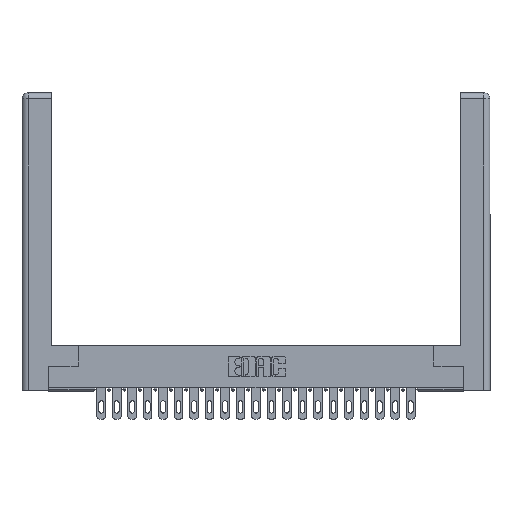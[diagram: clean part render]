
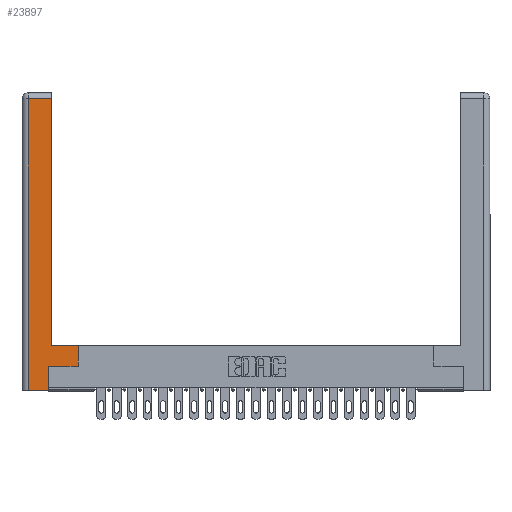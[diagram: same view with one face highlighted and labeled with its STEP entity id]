
A CAD part, top view. The second image highlights one B-rep face of the part: STEP entity #23897.
In plain terms, the highlighted planar face has unit normal (0, 0, 1).
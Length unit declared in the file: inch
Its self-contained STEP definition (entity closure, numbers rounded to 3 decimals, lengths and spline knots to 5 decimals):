
#56 = VERTEX_POINT ( 'NONE', #20512 ) ;
#331 = VERTEX_POINT ( 'NONE', #8046 ) ;
#447 = CARTESIAN_POINT ( 'NONE',  ( 0.565, 0.45, 0. ) ) ;
#482 = DIRECTION ( 'NONE',  ( 1., 0., 0. ) ) ;
#1216 = LINE ( 'NONE', #9743, #21261 ) ;
#1242 = CARTESIAN_POINT ( 'NONE',  ( 0.0615, 0., 0. ) ) ;
#1908 = EDGE_CURVE ( 'NONE', #331, #20292, #1216, .T. ) ;
#2259 = EDGE_CURVE ( 'NONE', #56, #16044, #23649, .T. ) ;
#2701 = DIRECTION ( 'NONE',  ( -1., 0., 0. ) ) ;
#2729 = CARTESIAN_POINT ( 'NONE',  ( 0.0615, 0., 0. ) ) ;
#3639 = EDGE_CURVE ( 'NONE', #20161, #331, #24363, .T. ) ;
#4570 = LINE ( 'NONE', #18500, #14320 ) ;
#4884 = DIRECTION ( 'NONE',  ( 0., 1., 0. ) ) ;
#5292 = DIRECTION ( 'NONE',  ( -1., 0., 0. ) ) ;
#5358 = CARTESIAN_POINT ( 'NONE',  ( 0.0615, 2.94, 0. ) ) ;
#5821 = DIRECTION ( 'NONE',  ( 1., 0., 0. ) ) ;
#6490 = EDGE_LOOP ( 'NONE', ( #11118, #15841, #23320, #9369, #12579, #12570, #23972, #16701 ) ) ;
#6543 = CARTESIAN_POINT ( 'NONE',  ( 0., 0., 0. ) ) ;
#7590 = AXIS2_PLACEMENT_3D ( 'NONE', #6543, #14395, #2701 ) ;
#7880 = VECTOR ( 'NONE', #23703, 39.37008 ) ;
#8046 = CARTESIAN_POINT ( 'NONE',  ( 0.265, 0., 0. ) ) ;
#8336 = VECTOR ( 'NONE', #5821, 39.37008 ) ;
#8548 = VECTOR ( 'NONE', #17423, 39.37008 ) ;
#8877 = EDGE_CURVE ( 'NONE', #19265, #56, #18883, .T. ) ;
#9369 = ORIENTED_EDGE ( 'NONE', *, *, #3639, .T. ) ;
#9617 = CARTESIAN_POINT ( 'NONE',  ( 0.295, 2.94, 0. ) ) ;
#9743 = CARTESIAN_POINT ( 'NONE',  ( 0.265, 0.245, 0. ) ) ;
#9927 = VECTOR ( 'NONE', #482, 39.37008 ) ;
#10900 = CARTESIAN_POINT ( 'NONE',  ( 0.265, 0.245, 0. ) ) ;
#11118 = ORIENTED_EDGE ( 'NONE', *, *, #20228, .T. ) ;
#12446 = PLANE ( 'NONE',  #7590 ) ;
#12570 = ORIENTED_EDGE ( 'NONE', *, *, #15140, .T. ) ;
#12579 = ORIENTED_EDGE ( 'NONE', *, *, #1908, .T. ) ;
#14009 = FACE_OUTER_BOUND ( 'NONE', #6490, .T. ) ;
#14320 = VECTOR ( 'NONE', #4884, 39.37008 ) ;
#14372 = DIRECTION ( 'NONE',  ( 0., 1., 0. ) ) ;
#14395 = DIRECTION ( 'NONE',  ( 0., 0., -1. ) ) ;
#14995 = VECTOR ( 'NONE', #18820, 39.37008 ) ;
#15140 = EDGE_CURVE ( 'NONE', #20292, #19265, #15175, .T. ) ;
#15175 = LINE ( 'NONE', #16152, #9927 ) ;
#15573 = CARTESIAN_POINT ( 'NONE',  ( 0.265, 0., 0. ) ) ;
#15841 = ORIENTED_EDGE ( 'NONE', *, *, #21684, .T. ) ;
#16044 = VERTEX_POINT ( 'NONE', #22467 ) ;
#16152 = CARTESIAN_POINT ( 'NONE',  ( 0.565, 0.245, 0. ) ) ;
#16474 = CARTESIAN_POINT ( 'NONE',  ( 0.295, 0.45, 0. ) ) ;
#16701 = ORIENTED_EDGE ( 'NONE', *, *, #2259, .T. ) ;
#16757 = VERTEX_POINT ( 'NONE', #9617 ) ;
#17423 = DIRECTION ( 'NONE',  ( -1., 0., 0. ) ) ;
#18500 = CARTESIAN_POINT ( 'NONE',  ( 0.295, 3., 0. ) ) ;
#18820 = DIRECTION ( 'NONE',  ( 0., -1., 0. ) ) ;
#18883 = LINE ( 'NONE', #447, #7880 ) ;
#19265 = VERTEX_POINT ( 'NONE', #22322 ) ;
#19343 = EDGE_CURVE ( 'NONE', #20952, #20161, #20702, .T. ) ;
#19356 = CARTESIAN_POINT ( 'NONE',  ( 0.0615, 2.94, 0. ) ) ;
#20161 = VERTEX_POINT ( 'NONE', #2729 ) ;
#20228 = EDGE_CURVE ( 'NONE', #16044, #16757, #4570, .T. ) ;
#20292 = VERTEX_POINT ( 'NONE', #10900 ) ;
#20512 = CARTESIAN_POINT ( 'NONE',  ( 0.565, 0.45, 0. ) ) ;
#20702 = LINE ( 'NONE', #1242, #14995 ) ;
#20952 = VERTEX_POINT ( 'NONE', #5358 ) ;
#21261 = VECTOR ( 'NONE', #14372, 39.37008 ) ;
#21684 = EDGE_CURVE ( 'NONE', #16757, #20952, #23985, .T. ) ;
#22322 = CARTESIAN_POINT ( 'NONE',  ( 0.565, 0.245, 0. ) ) ;
#22467 = CARTESIAN_POINT ( 'NONE',  ( 0.295, 0.45, 0. ) ) ;
#23053 = VECTOR ( 'NONE', #5292, 39.37008 ) ;
#23320 = ORIENTED_EDGE ( 'NONE', *, *, #19343, .T. ) ;
#23649 = LINE ( 'NONE', #16474, #23053 ) ;
#23703 = DIRECTION ( 'NONE',  ( 0., 1., 0. ) ) ;
#23897 = ADVANCED_FACE ( 'NONE', ( #14009 ), #12446, .F. ) ;
#23972 = ORIENTED_EDGE ( 'NONE', *, *, #8877, .T. ) ;
#23985 = LINE ( 'NONE', #19356, #8548 ) ;
#24363 = LINE ( 'NONE', #15573, #8336 ) ;
